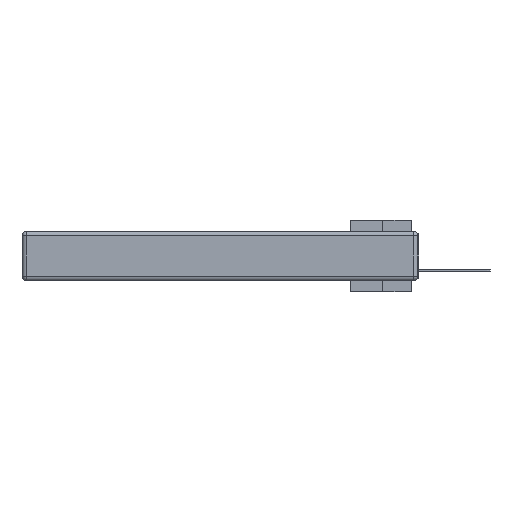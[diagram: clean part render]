
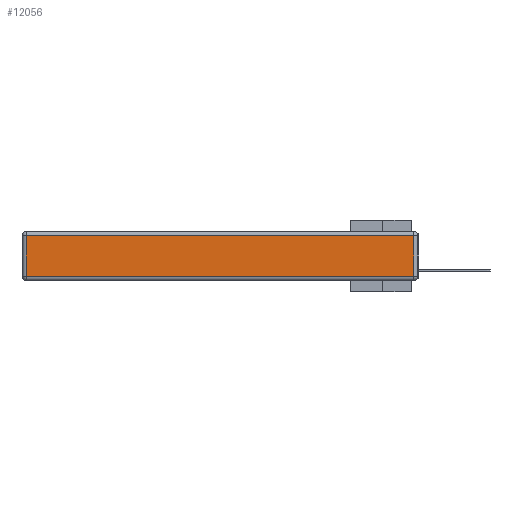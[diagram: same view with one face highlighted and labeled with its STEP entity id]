
A CAD part, left-side view. The second image highlights one B-rep face of the part: STEP entity #12056.
In plain terms, the highlighted planar face has unit normal (-1, 0, 0).
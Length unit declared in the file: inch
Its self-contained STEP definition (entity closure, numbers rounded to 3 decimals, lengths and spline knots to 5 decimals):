
#134 = VERTEX_POINT ( 'NONE', #10675 ) ;
#273 = ORIENTED_EDGE ( 'NONE', *, *, #8087, .T. ) ;
#601 = DIRECTION ( 'NONE',  ( 0., 0., 1. ) ) ;
#2367 = EDGE_CURVE ( 'NONE', #134, #13426, #8745, .T. ) ;
#2628 = CARTESIAN_POINT ( 'NONE',  ( 0., 2.72, -0.313 ) ) ;
#5932 = CARTESIAN_POINT ( 'NONE',  ( 0., 0., -0.343 ) ) ;
#6173 = DIRECTION ( 'NONE',  ( -1., 0., 0. ) ) ;
#6757 = VECTOR ( 'NONE', #601, 39.37008 ) ;
#7630 = LINE ( 'NONE', #26027, #25106 ) ;
#8087 = EDGE_CURVE ( 'NONE', #13426, #12106, #33482, .T. ) ;
#8745 = LINE ( 'NONE', #15857, #6757 ) ;
#10675 = CARTESIAN_POINT ( 'NONE',  ( 0., 0.03, -0.313 ) ) ;
#10805 = DIRECTION ( 'NONE',  ( 0., -1., 0. ) ) ;
#11849 = CARTESIAN_POINT ( 'NONE',  ( 0., 0.03, -0.03 ) ) ;
#12056 = ADVANCED_FACE ( 'NONE', ( #33336 ), #21696, .T. ) ;
#12106 = VERTEX_POINT ( 'NONE', #16852 ) ;
#12496 = CARTESIAN_POINT ( 'NONE',  ( 0., 2.75, -0.03 ) ) ;
#13426 = VERTEX_POINT ( 'NONE', #11849 ) ;
#15431 = ORIENTED_EDGE ( 'NONE', *, *, #26025, .T. ) ;
#15555 = VECTOR ( 'NONE', #20775, 39.37008 ) ;
#15857 = CARTESIAN_POINT ( 'NONE',  ( 0., 0.03, -0.343 ) ) ;
#16061 = VECTOR ( 'NONE', #29638, 39.37008 ) ;
#16077 = DIRECTION ( 'NONE',  ( 0., 0., 1. ) ) ;
#16852 = CARTESIAN_POINT ( 'NONE',  ( 0., 2.72, -0.03 ) ) ;
#20775 = DIRECTION ( 'NONE',  ( 0., 1., 0. ) ) ;
#21696 = PLANE ( 'NONE',  #23559 ) ;
#23559 = AXIS2_PLACEMENT_3D ( 'NONE', #5932, #6173, #16077 ) ;
#24709 = VERTEX_POINT ( 'NONE', #2628 ) ;
#25106 = VECTOR ( 'NONE', #10805, 39.37008 ) ;
#26025 = EDGE_CURVE ( 'NONE', #24709, #134, #7630, .T. ) ;
#26027 = CARTESIAN_POINT ( 'NONE',  ( 0., 0., -0.313 ) ) ;
#26722 = EDGE_LOOP ( 'NONE', ( #15431, #28679, #273, #32012 ) ) ;
#27372 = CARTESIAN_POINT ( 'NONE',  ( 0., 2.72, -0.343 ) ) ;
#28679 = ORIENTED_EDGE ( 'NONE', *, *, #2367, .T. ) ;
#29638 = DIRECTION ( 'NONE',  ( 0., 0., -1. ) ) ;
#29935 = LINE ( 'NONE', #27372, #16061 ) ;
#31564 = EDGE_CURVE ( 'NONE', #12106, #24709, #29935, .T. ) ;
#32012 = ORIENTED_EDGE ( 'NONE', *, *, #31564, .T. ) ;
#33336 = FACE_OUTER_BOUND ( 'NONE', #26722, .T. ) ;
#33482 = LINE ( 'NONE', #12496, #15555 ) ;
